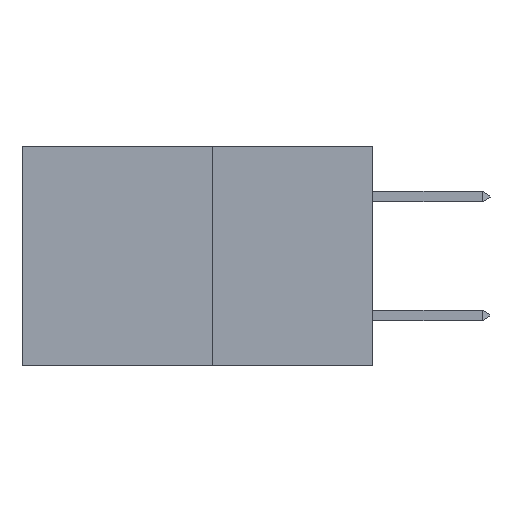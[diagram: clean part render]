
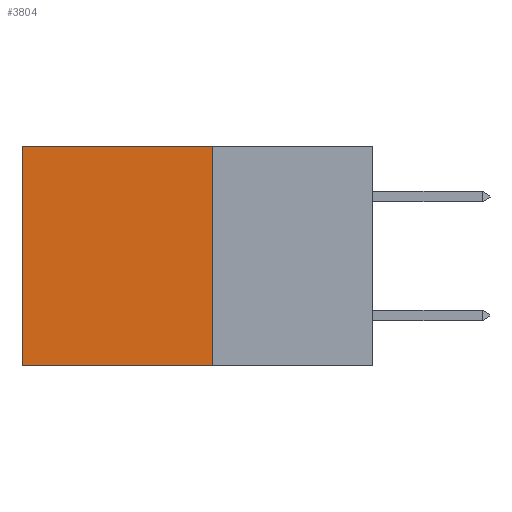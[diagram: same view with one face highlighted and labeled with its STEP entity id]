
A CAD part, left-side view. The second image highlights one B-rep face of the part: STEP entity #3804.
In plain terms, the highlighted planar face has unit normal (-1, 0, 0).
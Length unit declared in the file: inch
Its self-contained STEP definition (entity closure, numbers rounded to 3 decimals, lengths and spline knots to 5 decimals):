
#114 = DIRECTION ( 'NONE',  ( 0., 0., -1. ) ) ;
#588 = VECTOR ( 'NONE', #16870, 39.37008 ) ;
#818 = CARTESIAN_POINT ( 'NONE',  ( 0.277, 0.27, -0.37 ) ) ;
#1281 = ORIENTED_EDGE ( 'NONE', *, *, #17053, .T. ) ;
#2265 = VECTOR ( 'NONE', #114, 39.37008 ) ;
#2886 = CARTESIAN_POINT ( 'NONE',  ( 0.277, 0.59, 0. ) ) ;
#2947 = CARTESIAN_POINT ( 'NONE',  ( 0.277, 0.27, 0. ) ) ;
#3804 = ADVANCED_FACE ( 'NONE', ( #6514 ), #6216, .F. ) ;
#3973 = VERTEX_POINT ( 'NONE', #818 ) ;
#5191 = CARTESIAN_POINT ( 'NONE',  ( 0.277, 0.59, -0.37 ) ) ;
#5275 = DIRECTION ( 'NONE',  ( 0., 0., -1. ) ) ;
#5330 = DIRECTION ( 'NONE',  ( 1., 0., 0. ) ) ;
#5615 = CARTESIAN_POINT ( 'NONE',  ( 0.277, 0.27, -0.37 ) ) ;
#6216 = PLANE ( 'NONE',  #6852 ) ;
#6483 = LINE ( 'NONE', #16420, #18752 ) ;
#6514 = FACE_OUTER_BOUND ( 'NONE', #7468, .T. ) ;
#6552 = ORIENTED_EDGE ( 'NONE', *, *, #7715, .T. ) ;
#6852 = AXIS2_PLACEMENT_3D ( 'NONE', #5615, #5330, #5275 ) ;
#7291 = LINE ( 'NONE', #11959, #2265 ) ;
#7468 = EDGE_LOOP ( 'NONE', ( #6552, #20552, #15475, #1281 ) ) ;
#7715 = EDGE_CURVE ( 'NONE', #20810, #13519, #17878, .T. ) ;
#8175 = DIRECTION ( 'NONE',  ( 0., 1., 0. ) ) ;
#10683 = CARTESIAN_POINT ( 'NONE',  ( 0.277, 0.27, 0. ) ) ;
#10802 = CARTESIAN_POINT ( 'NONE',  ( 0.277, 0.59, -0.37 ) ) ;
#11959 = CARTESIAN_POINT ( 'NONE',  ( 0.277, 0.27, -0.37 ) ) ;
#12588 = EDGE_CURVE ( 'NONE', #3973, #13519, #6483, .T. ) ;
#12620 = LINE ( 'NONE', #2947, #18563 ) ;
#12773 = EDGE_CURVE ( 'NONE', #16249, #3973, #7291, .T. ) ;
#13519 = VERTEX_POINT ( 'NONE', #10802 ) ;
#14657 = DIRECTION ( 'NONE',  ( 0., 1., 0. ) ) ;
#15475 = ORIENTED_EDGE ( 'NONE', *, *, #12773, .F. ) ;
#16249 = VERTEX_POINT ( 'NONE', #10683 ) ;
#16420 = CARTESIAN_POINT ( 'NONE',  ( 0.277, 0.27, -0.37 ) ) ;
#16870 = DIRECTION ( 'NONE',  ( 0., 0., -1. ) ) ;
#17053 = EDGE_CURVE ( 'NONE', #16249, #20810, #12620, .T. ) ;
#17878 = LINE ( 'NONE', #5191, #588 ) ;
#18563 = VECTOR ( 'NONE', #14657, 39.37008 ) ;
#18752 = VECTOR ( 'NONE', #8175, 39.37008 ) ;
#20552 = ORIENTED_EDGE ( 'NONE', *, *, #12588, .F. ) ;
#20810 = VERTEX_POINT ( 'NONE', #2886 ) ;
